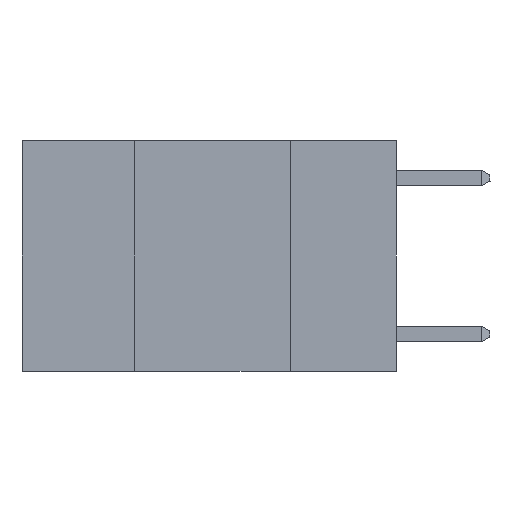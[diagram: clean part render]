
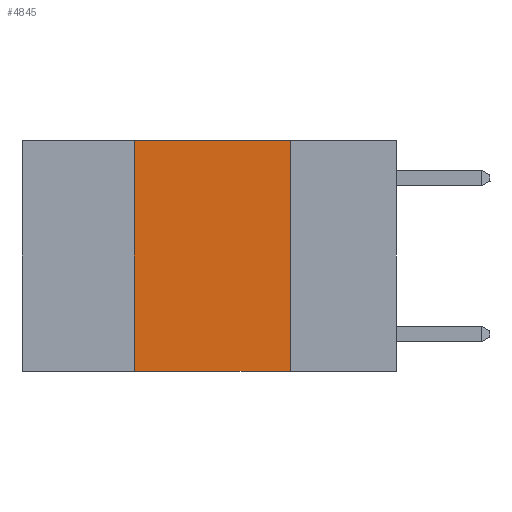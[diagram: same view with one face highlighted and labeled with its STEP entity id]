
A CAD part, left-side view. The second image highlights one B-rep face of the part: STEP entity #4845.
In plain terms, the highlighted planar face has unit normal (-1, 0, 0).
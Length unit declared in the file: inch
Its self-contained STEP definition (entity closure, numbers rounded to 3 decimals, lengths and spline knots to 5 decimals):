
#430 = CARTESIAN_POINT ( 'NONE',  ( 0., 0.6, 0. ) ) ;
#633 = ORIENTED_EDGE ( 'NONE', *, *, #7041, .F. ) ;
#1058 = EDGE_CURVE ( 'NONE', #15768, #14006, #9182, .T. ) ;
#1181 = CARTESIAN_POINT ( 'NONE',  ( 0., 0.17, -0.37 ) ) ;
#1490 = ORIENTED_EDGE ( 'NONE', *, *, #2640, .T. ) ;
#2114 = VERTEX_POINT ( 'NONE', #7301 ) ;
#2640 = EDGE_CURVE ( 'NONE', #15768, #14300, #7132, .T. ) ;
#3196 = CARTESIAN_POINT ( 'NONE',  ( 0., 0.17, 0. ) ) ;
#3541 = VECTOR ( 'NONE', #6012, 39.37008 ) ;
#4845 = ADVANCED_FACE ( 'NONE', ( #6901 ), #14700, .F. ) ;
#5994 = CARTESIAN_POINT ( 'NONE',  ( 0., 0.6, 0. ) ) ;
#6012 = DIRECTION ( 'NONE',  ( 0., -1., 0. ) ) ;
#6034 = CARTESIAN_POINT ( 'NONE',  ( 0., 0.6, -0.37 ) ) ;
#6402 = DIRECTION ( 'NONE',  ( 1., 0., 0. ) ) ;
#6901 = FACE_OUTER_BOUND ( 'NONE', #15624, .T. ) ;
#7041 = EDGE_CURVE ( 'NONE', #2114, #14300, #17727, .T. ) ;
#7132 = LINE ( 'NONE', #6034, #3541 ) ;
#7301 = CARTESIAN_POINT ( 'NONE',  ( 0., 0.17, 0. ) ) ;
#8188 = AXIS2_PLACEMENT_3D ( 'NONE', #430, #6402, #16093 ) ;
#8775 = DIRECTION ( 'NONE',  ( 0., -1., 0. ) ) ;
#9182 = LINE ( 'NONE', #14473, #12388 ) ;
#11708 = ORIENTED_EDGE ( 'NONE', *, *, #13883, .F. ) ;
#12388 = VECTOR ( 'NONE', #14535, 39.37008 ) ;
#13562 = CARTESIAN_POINT ( 'NONE',  ( 0., 0.42, -0.37 ) ) ;
#13883 = EDGE_CURVE ( 'NONE', #14006, #2114, #16184, .T. ) ;
#14006 = VERTEX_POINT ( 'NONE', #15889 ) ;
#14300 = VERTEX_POINT ( 'NONE', #1181 ) ;
#14473 = CARTESIAN_POINT ( 'NONE',  ( 0., 0.42, 0. ) ) ;
#14535 = DIRECTION ( 'NONE',  ( 0., 0., 1. ) ) ;
#14700 = PLANE ( 'NONE',  #8188 ) ;
#14964 = VECTOR ( 'NONE', #15936, 39.37008 ) ;
#15624 = EDGE_LOOP ( 'NONE', ( #633, #11708, #16209, #1490 ) ) ;
#15747 = VECTOR ( 'NONE', #8775, 39.37008 ) ;
#15768 = VERTEX_POINT ( 'NONE', #13562 ) ;
#15889 = CARTESIAN_POINT ( 'NONE',  ( 0., 0.42, 0. ) ) ;
#15936 = DIRECTION ( 'NONE',  ( 0., 0., -1. ) ) ;
#16093 = DIRECTION ( 'NONE',  ( 0., 0., -1. ) ) ;
#16184 = LINE ( 'NONE', #5994, #15747 ) ;
#16209 = ORIENTED_EDGE ( 'NONE', *, *, #1058, .F. ) ;
#17727 = LINE ( 'NONE', #3196, #14964 ) ;
